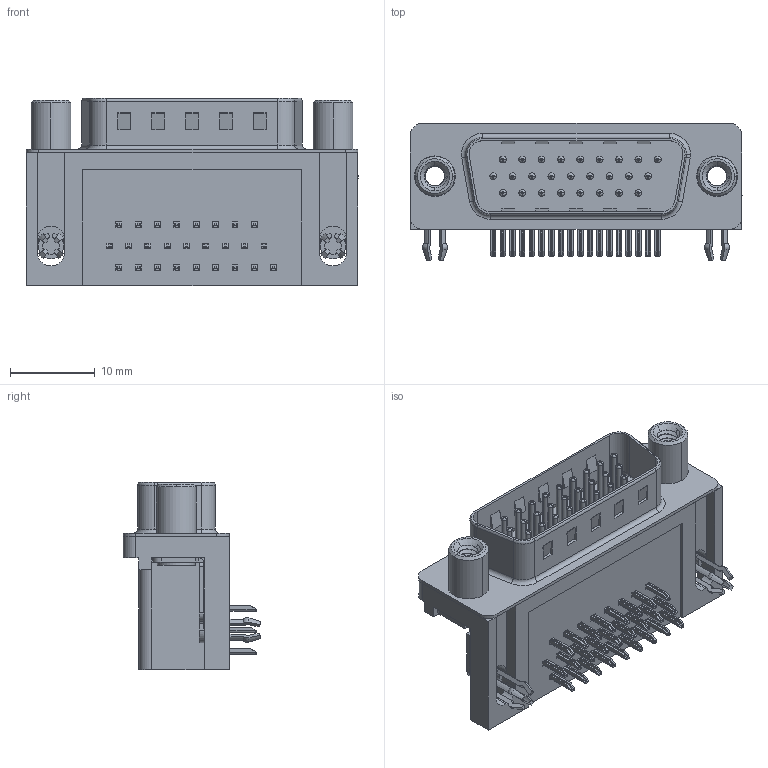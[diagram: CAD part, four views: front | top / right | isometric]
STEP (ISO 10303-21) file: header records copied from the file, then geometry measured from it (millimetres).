
FILE_DESCRIPTION (( 'STEP AP203' ), '1' );
FILE_NAME ('633-026-263-040.STEP', '2018-11-08T23:39:16', ( '' ), ( '' ), 'SwSTEP 2.0', 'SolidWorks 2016', '' );
FILE_SCHEMA (( 'CONFIG_CONTROL_DESIGN' ));
Length unit declared in the file: millimetre
Products named in the file (8): 633 Contact Bottom; 633 Contact Middle; 633 Contact Top; 633 4 Prong Board Lock; 633 Round Threaded Standoff; 633-026-263-040; 633 Housing_26 Contact; 633 Shell_26 Contact
Assembly tree (32 placements, depth 2):
  633-026-263-040
    633 Housing_26 Contact
    633 Shell_26 Contact
    633 Contact Bottom  x8
    633 Contact Middle  x9
    633 Contact Top  x9
    633 4 Prong Board Lock  x2
    633 Round Threaded Standoff  x2
Bounding box: 39.22 x 16.25 x 22.1 mm (x, y, z)
Volume: 5697.9 mm3; surface area: 7523.4 mm2
Topology: 32 solids, 32 shells, 2418 faces, 6054 edges, 3757 vertices
Faces by surface type: plane 1455, cylinder 692, torus 203, cone 52, bspline 16
Entity records: 25981 total; most frequent: CARTESIAN_POINT 5888, DIRECTION 3955, ORIENTED_EDGE 3796, EDGE_CURVE 1898, AXIS2_PLACEMENT_3D 1346, LINE 1263, VECTOR 1263, VERTEX_POINT 1219
